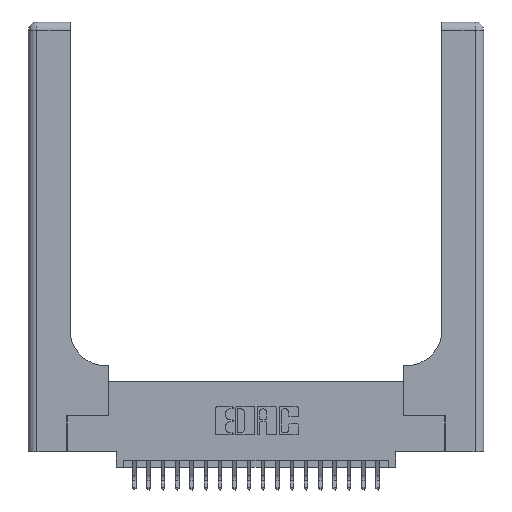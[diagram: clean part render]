
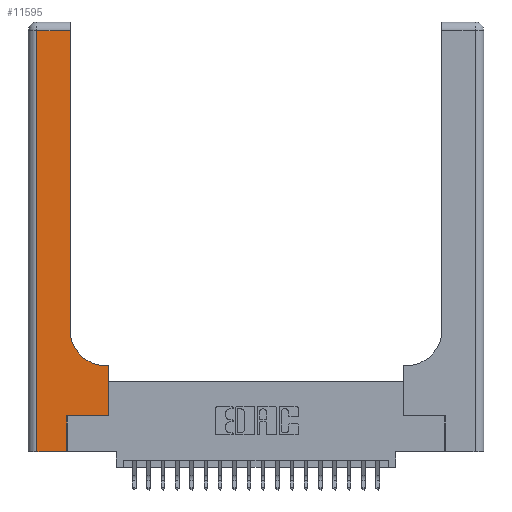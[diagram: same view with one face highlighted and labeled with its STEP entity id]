
A CAD part, top view. The second image highlights one B-rep face of the part: STEP entity #11595.
In plain terms, the highlighted planar face has unit normal (0, 0, 1).
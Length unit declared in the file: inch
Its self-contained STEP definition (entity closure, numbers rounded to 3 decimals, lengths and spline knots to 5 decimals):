
#169 = DIRECTION ( 'NONE',  ( 1., 0., 0. ) ) ;
#271 = CARTESIAN_POINT ( 'NONE',  ( 0.5585, 0.25, 0.37 ) ) ;
#710 = CARTESIAN_POINT ( 'NONE',  ( 0.5585, 0.25, 0.37 ) ) ;
#743 = VECTOR ( 'NONE', #788, 39.37008 ) ;
#788 = DIRECTION ( 'NONE',  ( 0., 1., 0. ) ) ;
#802 = VERTEX_POINT ( 'NONE', #12209 ) ;
#818 = CARTESIAN_POINT ( 'NONE',  ( 0.5415, 0.85, 0.37 ) ) ;
#1152 = DIRECTION ( 'NONE',  ( 0., 1., 0. ) ) ;
#1826 = ORIENTED_EDGE ( 'NONE', *, *, #7686, .T. ) ;
#2024 = DIRECTION ( 'NONE',  ( 0., 0., -1. ) ) ;
#2307 = DIRECTION ( 'NONE',  ( 0., 1., 0. ) ) ;
#2319 = CARTESIAN_POINT ( 'NONE',  ( 0.06, 3., 0.37 ) ) ;
#2361 = LINE ( 'NONE', #14301, #14833 ) ;
#2521 = LINE ( 'NONE', #710, #21816 ) ;
#2649 = DIRECTION ( 'NONE',  ( 1., 0., 0. ) ) ;
#3169 = LINE ( 'NONE', #3870, #12064 ) ;
#3765 = CARTESIAN_POINT ( 'NONE',  ( 0.269, 0.25, 0.37 ) ) ;
#3870 = CARTESIAN_POINT ( 'NONE',  ( 0., 0., 0.37 ) ) ;
#3937 = VERTEX_POINT ( 'NONE', #9936 ) ;
#3946 = VERTEX_POINT ( 'NONE', #4674 ) ;
#4007 = EDGE_CURVE ( 'NONE', #802, #5340, #13682, .T. ) ;
#4674 = CARTESIAN_POINT ( 'NONE',  ( 0.06, 2.94, 0.37 ) ) ;
#4998 = EDGE_CURVE ( 'NONE', #13440, #17338, #2521, .T. ) ;
#5340 = VERTEX_POINT ( 'NONE', #19805 ) ;
#5578 = LINE ( 'NONE', #13253, #743 ) ;
#5601 = CARTESIAN_POINT ( 'NONE',  ( 0., 3., 0.37 ) ) ;
#6232 = EDGE_CURVE ( 'NONE', #21954, #13440, #6867, .T. ) ;
#6867 = LINE ( 'NONE', #3765, #15664 ) ;
#7300 = DIRECTION ( 'NONE',  ( -1., 0., 0. ) ) ;
#7612 = CARTESIAN_POINT ( 'NONE',  ( 0., 2.94, 0.37 ) ) ;
#7622 = EDGE_CURVE ( 'NONE', #15249, #9454, #3169, .T. ) ;
#7686 = EDGE_CURVE ( 'NONE', #5340, #3946, #15055, .T. ) ;
#8116 = EDGE_CURVE ( 'NONE', #3946, #15249, #16139, .T. ) ;
#8225 = CARTESIAN_POINT ( 'NONE',  ( 0.269, 0., 0.37 ) ) ;
#8457 = VECTOR ( 'NONE', #1152, 39.37008 ) ;
#8694 = CARTESIAN_POINT ( 'NONE',  ( 0.5585, 0.6, 0.37 ) ) ;
#9396 = DIRECTION ( 'NONE',  ( -1., 0., 0. ) ) ;
#9454 = VERTEX_POINT ( 'NONE', #8225 ) ;
#9850 = ORIENTED_EDGE ( 'NONE', *, *, #4007, .T. ) ;
#9936 = CARTESIAN_POINT ( 'NONE',  ( 0.5415, 0.6, 0.37 ) ) ;
#9959 = ORIENTED_EDGE ( 'NONE', *, *, #8116, .T. ) ;
#10424 = VECTOR ( 'NONE', #9396, 39.37008 ) ;
#10495 = CARTESIAN_POINT ( 'NONE',  ( 0.269, 0.25, 0.37 ) ) ;
#10573 = EDGE_CURVE ( 'NONE', #9454, #21954, #5578, .T. ) ;
#10937 = VECTOR ( 'NONE', #16560, 39.37008 ) ;
#11595 = ADVANCED_FACE ( 'NONE', ( #17654 ), #12700, .F. ) ;
#12064 = VECTOR ( 'NONE', #16215, 39.37008 ) ;
#12209 = CARTESIAN_POINT ( 'NONE',  ( 0.2915, 0.85, 0.37 ) ) ;
#12700 = PLANE ( 'NONE',  #20179 ) ;
#13099 = ORIENTED_EDGE ( 'NONE', *, *, #6232, .T. ) ;
#13253 = CARTESIAN_POINT ( 'NONE',  ( 0.269, 0., 0.37 ) ) ;
#13283 = DIRECTION ( 'NONE',  ( 0., 0., -1. ) ) ;
#13440 = VERTEX_POINT ( 'NONE', #271 ) ;
#13451 = ORIENTED_EDGE ( 'NONE', *, *, #20208, .T. ) ;
#13562 = CIRCLE ( 'NONE', #14959, 0.25 ) ;
#13682 = LINE ( 'NONE', #20558, #8457 ) ;
#14301 = CARTESIAN_POINT ( 'NONE',  ( 0.2915, 0.6, 0.37 ) ) ;
#14447 = DIRECTION ( 'NONE',  ( -1., 0., 0. ) ) ;
#14833 = VECTOR ( 'NONE', #7300, 39.37008 ) ;
#14959 = AXIS2_PLACEMENT_3D ( 'NONE', #818, #13283, #2649 ) ;
#15000 = ORIENTED_EDGE ( 'NONE', *, *, #10573, .T. ) ;
#15055 = LINE ( 'NONE', #7612, #10424 ) ;
#15249 = VERTEX_POINT ( 'NONE', #22679 ) ;
#15610 = EDGE_CURVE ( 'NONE', #3937, #802, #13562, .T. ) ;
#15630 = ORIENTED_EDGE ( 'NONE', *, *, #15610, .T. ) ;
#15664 = VECTOR ( 'NONE', #169, 39.37008 ) ;
#16139 = LINE ( 'NONE', #2319, #10937 ) ;
#16215 = DIRECTION ( 'NONE',  ( 1., 0., 0. ) ) ;
#16560 = DIRECTION ( 'NONE',  ( 0., -1., 0. ) ) ;
#17338 = VERTEX_POINT ( 'NONE', #8694 ) ;
#17654 = FACE_OUTER_BOUND ( 'NONE', #22825, .T. ) ;
#19805 = CARTESIAN_POINT ( 'NONE',  ( 0.2915, 2.94, 0.37 ) ) ;
#20179 = AXIS2_PLACEMENT_3D ( 'NONE', #5601, #2024, #14447 ) ;
#20208 = EDGE_CURVE ( 'NONE', #17338, #3937, #2361, .T. ) ;
#20483 = ORIENTED_EDGE ( 'NONE', *, *, #4998, .T. ) ;
#20558 = CARTESIAN_POINT ( 'NONE',  ( 0.2915, 3., 0.37 ) ) ;
#21816 = VECTOR ( 'NONE', #2307, 39.37008 ) ;
#21954 = VERTEX_POINT ( 'NONE', #10495 ) ;
#22528 = ORIENTED_EDGE ( 'NONE', *, *, #7622, .T. ) ;
#22679 = CARTESIAN_POINT ( 'NONE',  ( 0.06, 0., 0.37 ) ) ;
#22825 = EDGE_LOOP ( 'NONE', ( #9850, #1826, #9959, #22528, #15000, #13099, #20483, #13451, #15630 ) ) ;
